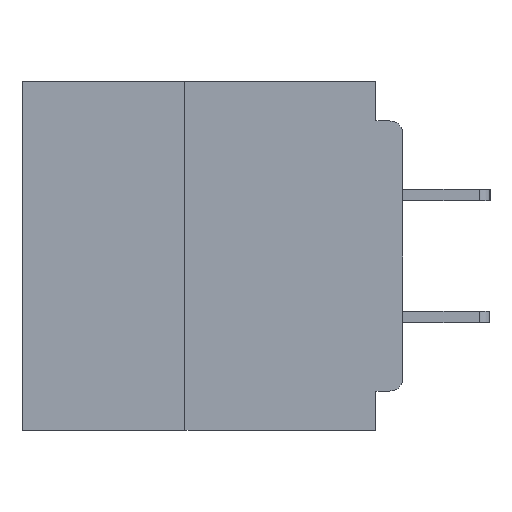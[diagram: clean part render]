
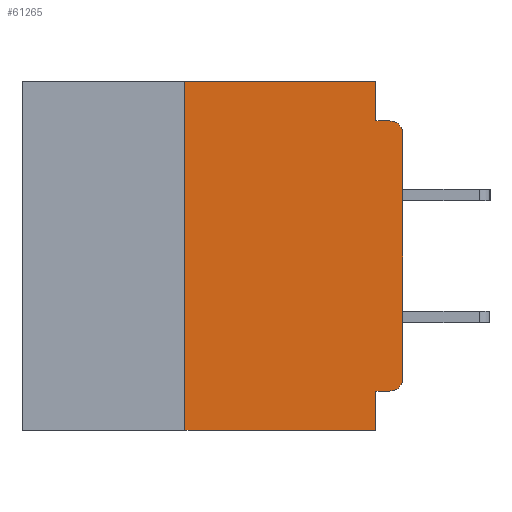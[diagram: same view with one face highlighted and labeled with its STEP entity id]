
A CAD part, left-side view. The second image highlights one B-rep face of the part: STEP entity #61265.
In plain terms, the highlighted planar face has unit normal (-1, 0, 0).
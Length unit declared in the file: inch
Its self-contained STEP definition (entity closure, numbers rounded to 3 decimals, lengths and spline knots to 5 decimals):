
#460 = VECTOR ( 'NONE', #12086, 39.37008 ) ;
#1132 = VECTOR ( 'NONE', #21894, 39.37008 ) ;
#1232 = DIRECTION ( 'NONE',  ( 0., 0., -1. ) ) ;
#1881 = CARTESIAN_POINT ( 'NONE',  ( 0., 0.437, 0. ) ) ;
#2578 = CIRCLE ( 'NONE', #18283, 0.015 ) ;
#3002 = ORIENTED_EDGE ( 'NONE', *, *, #59668, .T. ) ;
#3169 = DIRECTION ( 'NONE',  ( 0., 0., -1. ) ) ;
#5628 = CARTESIAN_POINT ( 'NONE',  ( 0., 0., 0. ) ) ;
#5796 = LINE ( 'NONE', #1881, #55262 ) ;
#7517 = ORIENTED_EDGE ( 'NONE', *, *, #28956, .F. ) ;
#7869 = AXIS2_PLACEMENT_3D ( 'NONE', #22306, #31924, #3169 ) ;
#8003 = VERTEX_POINT ( 'NONE', #49816 ) ;
#8244 = CARTESIAN_POINT ( 'NONE',  ( 0., 0.437, -0.4 ) ) ;
#9324 = CARTESIAN_POINT ( 'NONE',  ( 0., 0.031, -0.4 ) ) ;
#9361 = VERTEX_POINT ( 'NONE', #13846 ) ;
#9405 = VERTEX_POINT ( 'NONE', #47789 ) ;
#10386 = EDGE_CURVE ( 'NONE', #29114, #48637, #39462, .T. ) ;
#10945 = CARTESIAN_POINT ( 'NONE',  ( 0., 0.031, -0.045 ) ) ;
#11188 = AXIS2_PLACEMENT_3D ( 'NONE', #18255, #51712, #23079 ) ;
#11465 = ORIENTED_EDGE ( 'NONE', *, *, #61727, .F. ) ;
#12086 = DIRECTION ( 'NONE',  ( 0., 1., 0. ) ) ;
#13247 = LINE ( 'NONE', #26398, #460 ) ;
#13414 = CARTESIAN_POINT ( 'NONE',  ( 0., 0.015, -0.06 ) ) ;
#13846 = CARTESIAN_POINT ( 'NONE',  ( 0., 0., -0.06 ) ) ;
#14646 = VERTEX_POINT ( 'NONE', #21910 ) ;
#15174 = EDGE_CURVE ( 'NONE', #9405, #26069, #5796, .T. ) ;
#17736 = EDGE_CURVE ( 'NONE', #31587, #24884, #13247, .T. ) ;
#18214 = FACE_OUTER_BOUND ( 'NONE', #58825, .T. ) ;
#18229 = ORIENTED_EDGE ( 'NONE', *, *, #15174, .F. ) ;
#18255 = CARTESIAN_POINT ( 'NONE',  ( 0., 0.015, -0.34 ) ) ;
#18258 = DIRECTION ( 'NONE',  ( 0., 0., -1. ) ) ;
#18283 = AXIS2_PLACEMENT_3D ( 'NONE', #13414, #46958, #18258 ) ;
#20949 = VECTOR ( 'NONE', #48328, 39.37008 ) ;
#21152 = ORIENTED_EDGE ( 'NONE', *, *, #54626, .T. ) ;
#21894 = DIRECTION ( 'NONE',  ( 0., -1., 0. ) ) ;
#21910 = CARTESIAN_POINT ( 'NONE',  ( 0., 0.25, -0.4 ) ) ;
#22306 = CARTESIAN_POINT ( 'NONE',  ( 0., 0.437, 0. ) ) ;
#23079 = DIRECTION ( 'NONE',  ( 0., 0., -1. ) ) ;
#23715 = VECTOR ( 'NONE', #48874, 39.37008 ) ;
#24670 = VERTEX_POINT ( 'NONE', #9324 ) ;
#24884 = VERTEX_POINT ( 'NONE', #25704 ) ;
#25704 = CARTESIAN_POINT ( 'NONE',  ( 0., 0.031, -0.355 ) ) ;
#25786 = ORIENTED_EDGE ( 'NONE', *, *, #17736, .F. ) ;
#26069 = VERTEX_POINT ( 'NONE', #30997 ) ;
#26398 = CARTESIAN_POINT ( 'NONE',  ( 0., 0., -0.355 ) ) ;
#28956 = EDGE_CURVE ( 'NONE', #26069, #29114, #36169, .T. ) ;
#29114 = VERTEX_POINT ( 'NONE', #10945 ) ;
#30897 = LINE ( 'NONE', #34825, #56302 ) ;
#30997 = CARTESIAN_POINT ( 'NONE',  ( 0., 0.031, 0. ) ) ;
#31587 = VERTEX_POINT ( 'NONE', #42636 ) ;
#31924 = DIRECTION ( 'NONE',  ( 1., 0., 0. ) ) ;
#32113 = ORIENTED_EDGE ( 'NONE', *, *, #45270, .T. ) ;
#32403 = DIRECTION ( 'NONE',  ( 0., -1., 0. ) ) ;
#33860 = CARTESIAN_POINT ( 'NONE',  ( 0., 0.031, 0. ) ) ;
#34825 = CARTESIAN_POINT ( 'NONE',  ( 0., 0.031, -0.4 ) ) ;
#36169 = LINE ( 'NONE', #33860, #47410 ) ;
#38153 = ORIENTED_EDGE ( 'NONE', *, *, #10386, .F. ) ;
#38694 = DIRECTION ( 'NONE',  ( 0., 0., -1. ) ) ;
#39462 = LINE ( 'NONE', #55305, #1132 ) ;
#40342 = EDGE_CURVE ( 'NONE', #14646, #9405, #46428, .T. ) ;
#41119 = ORIENTED_EDGE ( 'NONE', *, *, #40342, .F. ) ;
#41387 = PLANE ( 'NONE',  #7869 ) ;
#42027 = ORIENTED_EDGE ( 'NONE', *, *, #60040, .T. ) ;
#42636 = CARTESIAN_POINT ( 'NONE',  ( 0., 0.015, -0.355 ) ) ;
#43523 = CARTESIAN_POINT ( 'NONE',  ( 0., 0.25, -0.4 ) ) ;
#45093 = DIRECTION ( 'NONE',  ( 0., -1., 0. ) ) ;
#45270 = EDGE_CURVE ( 'NONE', #14646, #24670, #56303, .T. ) ;
#46428 = LINE ( 'NONE', #43523, #20949 ) ;
#46958 = DIRECTION ( 'NONE',  ( -1., 0., 0. ) ) ;
#47410 = VECTOR ( 'NONE', #38694, 39.37008 ) ;
#47789 = CARTESIAN_POINT ( 'NONE',  ( 0., 0.25, 0. ) ) ;
#48046 = CIRCLE ( 'NONE', #11188, 0.015 ) ;
#48328 = DIRECTION ( 'NONE',  ( 0., 0., 1. ) ) ;
#48637 = VERTEX_POINT ( 'NONE', #52969 ) ;
#48874 = DIRECTION ( 'NONE',  ( 0., 0., 1. ) ) ;
#49157 = LINE ( 'NONE', #5628, #23715 ) ;
#49816 = CARTESIAN_POINT ( 'NONE',  ( 0., 0., -0.34 ) ) ;
#51712 = DIRECTION ( 'NONE',  ( -1., 0., 0. ) ) ;
#52969 = CARTESIAN_POINT ( 'NONE',  ( 0., 0.015, -0.045 ) ) ;
#54626 = EDGE_CURVE ( 'NONE', #31587, #8003, #48046, .T. ) ;
#55262 = VECTOR ( 'NONE', #45093, 39.37008 ) ;
#55305 = CARTESIAN_POINT ( 'NONE',  ( 0., 0., -0.045 ) ) ;
#56302 = VECTOR ( 'NONE', #1232, 39.37008 ) ;
#56303 = LINE ( 'NONE', #8244, #57813 ) ;
#57813 = VECTOR ( 'NONE', #32403, 39.37008 ) ;
#58825 = EDGE_LOOP ( 'NONE', ( #3002, #42027, #38153, #7517, #18229, #41119, #32113, #11465, #25786, #21152 ) ) ;
#59668 = EDGE_CURVE ( 'NONE', #8003, #9361, #49157, .T. ) ;
#60040 = EDGE_CURVE ( 'NONE', #9361, #48637, #2578, .T. ) ;
#61265 = ADVANCED_FACE ( 'NONE', ( #18214 ), #41387, .F. ) ;
#61727 = EDGE_CURVE ( 'NONE', #24884, #24670, #30897, .T. ) ;
